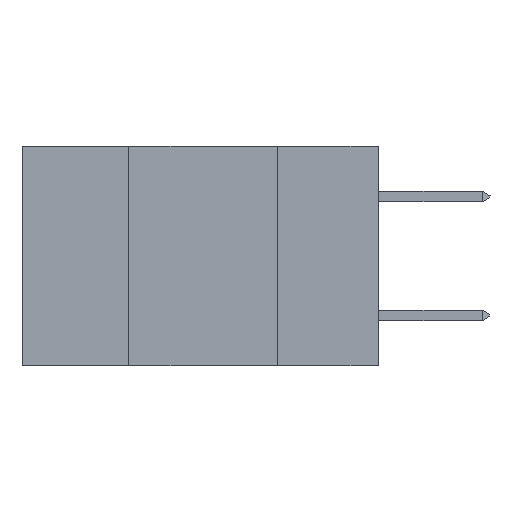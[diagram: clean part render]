
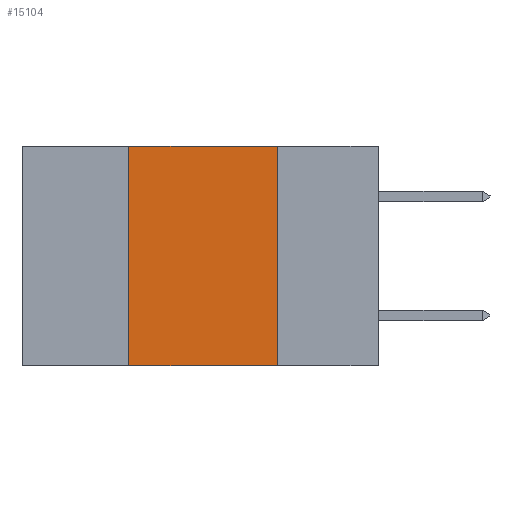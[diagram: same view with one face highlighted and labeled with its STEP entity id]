
A CAD part, left-side view. The second image highlights one B-rep face of the part: STEP entity #15104.
In plain terms, the highlighted planar face has unit normal (-1, 0, 0).
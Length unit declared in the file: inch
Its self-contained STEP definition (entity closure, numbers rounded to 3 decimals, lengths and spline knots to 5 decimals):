
#937 = DIRECTION ( 'NONE',  ( 0., -1., 0. ) ) ;
#1160 = CARTESIAN_POINT ( 'NONE',  ( 0., 0.6, 0. ) ) ;
#1407 = EDGE_CURVE ( 'NONE', #6364, #15997, #11463, .T. ) ;
#2234 = CARTESIAN_POINT ( 'NONE',  ( 0., 0.17, -0.37 ) ) ;
#2323 = DIRECTION ( 'NONE',  ( 0., 0., -1. ) ) ;
#2997 = CARTESIAN_POINT ( 'NONE',  ( 0., 0.17, -0.37 ) ) ;
#3116 = CARTESIAN_POINT ( 'NONE',  ( 0., 0.6, 0. ) ) ;
#3232 = VECTOR ( 'NONE', #937, 39.37008 ) ;
#3426 = LINE ( 'NONE', #3116, #13985 ) ;
#4183 = EDGE_CURVE ( 'NONE', #16669, #15997, #18083, .T. ) ;
#4853 = ORIENTED_EDGE ( 'NONE', *, *, #1407, .F. ) ;
#5105 = CARTESIAN_POINT ( 'NONE',  ( 0., 0.17, 0. ) ) ;
#5695 = VECTOR ( 'NONE', #14737, 39.37008 ) ;
#6364 = VERTEX_POINT ( 'NONE', #5105 ) ;
#8618 = ORIENTED_EDGE ( 'NONE', *, *, #18156, .F. ) ;
#8869 = FACE_OUTER_BOUND ( 'NONE', #16263, .T. ) ;
#10740 = AXIS2_PLACEMENT_3D ( 'NONE', #1160, #17901, #2323 ) ;
#11109 = DIRECTION ( 'NONE',  ( 0., -1., 0. ) ) ;
#11463 = LINE ( 'NONE', #2234, #5695 ) ;
#11877 = DIRECTION ( 'NONE',  ( 0., 0., 1. ) ) ;
#12894 = CARTESIAN_POINT ( 'NONE',  ( 0., 0.42, -0.37 ) ) ;
#13985 = VECTOR ( 'NONE', #11109, 39.37008 ) ;
#14262 = EDGE_CURVE ( 'NONE', #14485, #6364, #3426, .T. ) ;
#14485 = VERTEX_POINT ( 'NONE', #16848 ) ;
#14737 = DIRECTION ( 'NONE',  ( 0., 0., -1. ) ) ;
#14948 = LINE ( 'NONE', #19679, #18886 ) ;
#15104 = ADVANCED_FACE ( 'NONE', ( #8869 ), #15140, .F. ) ;
#15140 = PLANE ( 'NONE',  #10740 ) ;
#15997 = VERTEX_POINT ( 'NONE', #2997 ) ;
#16263 = EDGE_LOOP ( 'NONE', ( #4853, #16553, #8618, #16502 ) ) ;
#16502 = ORIENTED_EDGE ( 'NONE', *, *, #4183, .T. ) ;
#16553 = ORIENTED_EDGE ( 'NONE', *, *, #14262, .F. ) ;
#16669 = VERTEX_POINT ( 'NONE', #12894 ) ;
#16848 = CARTESIAN_POINT ( 'NONE',  ( 0., 0.42, 0. ) ) ;
#17901 = DIRECTION ( 'NONE',  ( 1., 0., 0. ) ) ;
#18083 = LINE ( 'NONE', #18380, #3232 ) ;
#18156 = EDGE_CURVE ( 'NONE', #16669, #14485, #14948, .T. ) ;
#18380 = CARTESIAN_POINT ( 'NONE',  ( 0., 0.6, -0.37 ) ) ;
#18886 = VECTOR ( 'NONE', #11877, 39.37008 ) ;
#19679 = CARTESIAN_POINT ( 'NONE',  ( 0., 0.42, -0.37 ) ) ;
